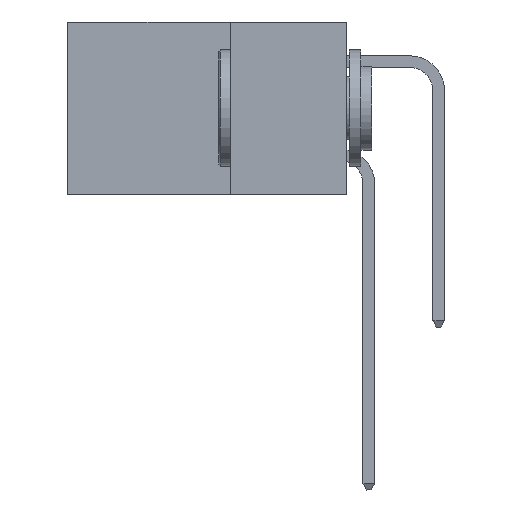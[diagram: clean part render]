
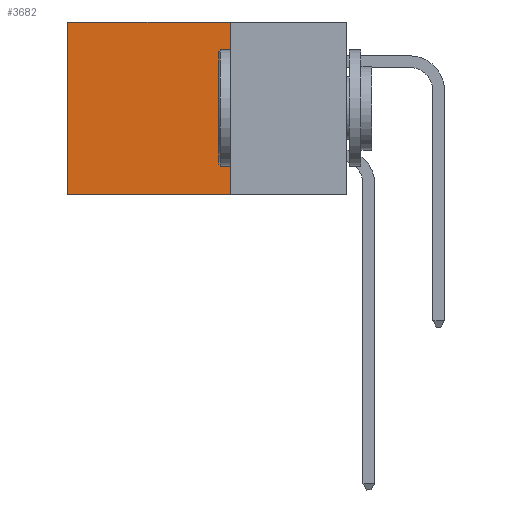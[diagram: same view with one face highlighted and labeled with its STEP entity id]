
A CAD part, left-side view. The second image highlights one B-rep face of the part: STEP entity #3682.
In plain terms, the highlighted planar face has unit normal (-1, 0, 0).
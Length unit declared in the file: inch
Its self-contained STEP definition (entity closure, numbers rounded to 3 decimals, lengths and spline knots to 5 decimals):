
#681 = DIRECTION ( 'NONE',  ( 0., 1., 0. ) ) ;
#881 = EDGE_CURVE ( 'NONE', #15745, #12018, #9111, .T. ) ;
#1560 = VECTOR ( 'NONE', #2928, 39.37008 ) ;
#2439 = CARTESIAN_POINT ( 'NONE',  ( 0.2875, 0.25, -0.37 ) ) ;
#2487 = PLANE ( 'NONE',  #10432 ) ;
#2490 = DIRECTION ( 'NONE',  ( 0., 0., -1. ) ) ;
#2556 = FACE_OUTER_BOUND ( 'NONE', #6107, .T. ) ;
#2667 = VERTEX_POINT ( 'NONE', #8647 ) ;
#2928 = DIRECTION ( 'NONE',  ( 0., 1., 0. ) ) ;
#3682 = ADVANCED_FACE ( 'NONE', ( #2556 ), #2487, .F. ) ;
#3880 = CARTESIAN_POINT ( 'NONE',  ( 0.2875, 0.25, 0. ) ) ;
#3938 = DIRECTION ( 'NONE',  ( 0., 0., -1. ) ) ;
#5496 = VECTOR ( 'NONE', #16759, 39.37008 ) ;
#5566 = ORIENTED_EDGE ( 'NONE', *, *, #11143, .F. ) ;
#6107 = EDGE_LOOP ( 'NONE', ( #8439, #5566, #14420, #14331 ) ) ;
#7377 = VECTOR ( 'NONE', #2490, 39.37008 ) ;
#8439 = ORIENTED_EDGE ( 'NONE', *, *, #16366, .T. ) ;
#8647 = CARTESIAN_POINT ( 'NONE',  ( 0.2875, 0.6, -0.37 ) ) ;
#8875 = CARTESIAN_POINT ( 'NONE',  ( 0.2875, 0.6, 0. ) ) ;
#9111 = LINE ( 'NONE', #14341, #1560 ) ;
#9543 = CARTESIAN_POINT ( 'NONE',  ( 0.2875, 0.25, 0. ) ) ;
#10432 = AXIS2_PLACEMENT_3D ( 'NONE', #3880, #12179, #3938 ) ;
#10874 = CARTESIAN_POINT ( 'NONE',  ( 0.2875, 0.6, 0. ) ) ;
#10972 = LINE ( 'NONE', #9543, #7377 ) ;
#11143 = EDGE_CURVE ( 'NONE', #14216, #2667, #16161, .T. ) ;
#12018 = VERTEX_POINT ( 'NONE', #10874 ) ;
#12179 = DIRECTION ( 'NONE',  ( 1., 0., 0. ) ) ;
#12653 = VECTOR ( 'NONE', #681, 39.37008 ) ;
#13114 = LINE ( 'NONE', #8875, #5496 ) ;
#13120 = CARTESIAN_POINT ( 'NONE',  ( 0.2875, 0.25, -0.37 ) ) ;
#14216 = VERTEX_POINT ( 'NONE', #2439 ) ;
#14331 = ORIENTED_EDGE ( 'NONE', *, *, #881, .T. ) ;
#14341 = CARTESIAN_POINT ( 'NONE',  ( 0.2875, 0.25, 0. ) ) ;
#14420 = ORIENTED_EDGE ( 'NONE', *, *, #17315, .F. ) ;
#15745 = VERTEX_POINT ( 'NONE', #16655 ) ;
#16161 = LINE ( 'NONE', #13120, #12653 ) ;
#16366 = EDGE_CURVE ( 'NONE', #12018, #2667, #13114, .T. ) ;
#16655 = CARTESIAN_POINT ( 'NONE',  ( 0.2875, 0.25, 0. ) ) ;
#16759 = DIRECTION ( 'NONE',  ( 0., 0., -1. ) ) ;
#17315 = EDGE_CURVE ( 'NONE', #15745, #14216, #10972, .T. ) ;
